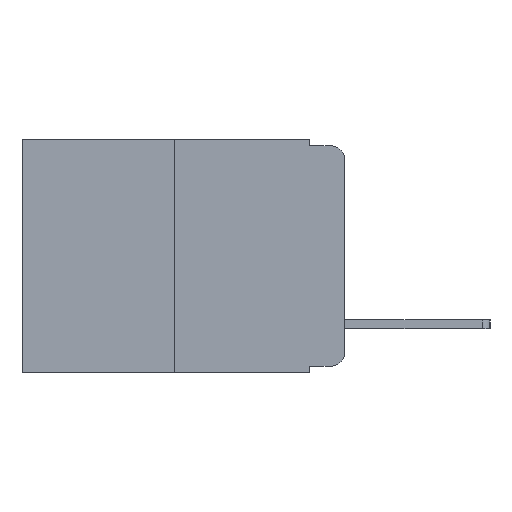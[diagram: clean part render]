
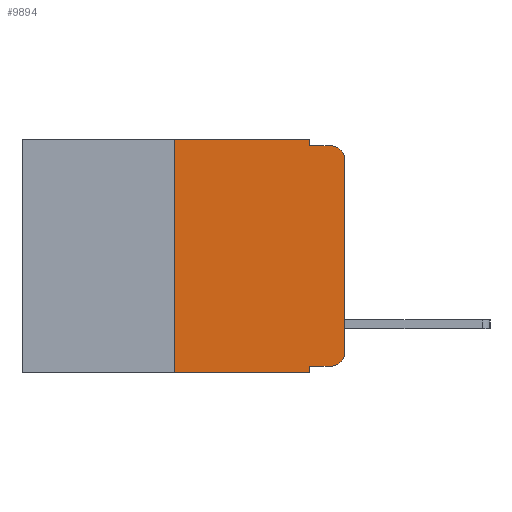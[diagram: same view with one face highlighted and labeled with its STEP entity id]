
A CAD part, left-side view. The second image highlights one B-rep face of the part: STEP entity #9894.
In plain terms, the highlighted planar face has unit normal (-1, 0, 0).
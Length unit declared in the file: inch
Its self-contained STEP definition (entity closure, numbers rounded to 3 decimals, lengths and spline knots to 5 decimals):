
#180 = ORIENTED_EDGE ( 'NONE', *, *, #7223, .T. ) ;
#393 = VERTEX_POINT ( 'NONE', #1976 ) ;
#436 = DIRECTION ( 'NONE',  ( -1., 0., 0. ) ) ;
#718 = CARTESIAN_POINT ( 'NONE',  ( 0., 0.25, 0. ) ) ;
#937 = AXIS2_PLACEMENT_3D ( 'NONE', #10834, #11770, #6180 ) ;
#984 = ORIENTED_EDGE ( 'NONE', *, *, #8508, .F. ) ;
#1038 = EDGE_CURVE ( 'NONE', #7669, #5206, #10918, .T. ) ;
#1183 = DIRECTION ( 'NONE',  ( 0., -1., 0. ) ) ;
#1198 = CARTESIAN_POINT ( 'NONE',  ( 0., 0.051, -0.01 ) ) ;
#1281 = DIRECTION ( 'NONE',  ( 0., -1., 0. ) ) ;
#1392 = LINE ( 'NONE', #8974, #8864 ) ;
#1441 = CARTESIAN_POINT ( 'NONE',  ( 0., 0.473, 0. ) ) ;
#1643 = DIRECTION ( 'NONE',  ( 0., 0., 1. ) ) ;
#1976 = CARTESIAN_POINT ( 'NONE',  ( 0., 0., -0.03 ) ) ;
#2035 = CARTESIAN_POINT ( 'NONE',  ( 0., 0.051, -0.01 ) ) ;
#2045 = VERTEX_POINT ( 'NONE', #6982 ) ;
#2068 = VERTEX_POINT ( 'NONE', #4722 ) ;
#2250 = ORIENTED_EDGE ( 'NONE', *, *, #1038, .F. ) ;
#2287 = ORIENTED_EDGE ( 'NONE', *, *, #7891, .T. ) ;
#2436 = EDGE_CURVE ( 'NONE', #393, #5206, #3619, .T. ) ;
#2439 = ORIENTED_EDGE ( 'NONE', *, *, #9096, .F. ) ;
#2883 = DIRECTION ( 'NONE',  ( 0., -1., 0. ) ) ;
#3076 = VECTOR ( 'NONE', #1183, 39.37008 ) ;
#3100 = EDGE_CURVE ( 'NONE', #3775, #393, #9310, .T. ) ;
#3619 = CIRCLE ( 'NONE', #5348, 0.02 ) ;
#3775 = VERTEX_POINT ( 'NONE', #7620 ) ;
#3866 = ORIENTED_EDGE ( 'NONE', *, *, #3100, .T. ) ;
#3903 = DIRECTION ( 'NONE',  ( 0., 0., -1. ) ) ;
#3988 = ORIENTED_EDGE ( 'NONE', *, *, #10944, .F. ) ;
#4083 = ORIENTED_EDGE ( 'NONE', *, *, #4863, .F. ) ;
#4165 = LINE ( 'NONE', #11394, #8971 ) ;
#4176 = ORIENTED_EDGE ( 'NONE', *, *, #11501, .T. ) ;
#4252 = ORIENTED_EDGE ( 'NONE', *, *, #2436, .T. ) ;
#4592 = VERTEX_POINT ( 'NONE', #7899 ) ;
#4722 = CARTESIAN_POINT ( 'NONE',  ( 0., 0.25, 0. ) ) ;
#4732 = CARTESIAN_POINT ( 'NONE',  ( 0., 0.473, -0.343 ) ) ;
#4863 = EDGE_CURVE ( 'NONE', #2068, #7177, #11222, .T. ) ;
#4869 = VECTOR ( 'NONE', #3903, 39.37008 ) ;
#5171 = PLANE ( 'NONE',  #937 ) ;
#5206 = VERTEX_POINT ( 'NONE', #6842 ) ;
#5252 = CARTESIAN_POINT ( 'NONE',  ( 0., 0.02, -0.313 ) ) ;
#5348 = AXIS2_PLACEMENT_3D ( 'NONE', #6390, #436, #7385 ) ;
#6058 = AXIS2_PLACEMENT_3D ( 'NONE', #5252, #11837, #6245 ) ;
#6180 = DIRECTION ( 'NONE',  ( 0., 0., -1. ) ) ;
#6240 = VECTOR ( 'NONE', #8288, 39.37008 ) ;
#6245 = DIRECTION ( 'NONE',  ( 0., 0., -1. ) ) ;
#6390 = CARTESIAN_POINT ( 'NONE',  ( 0., 0.02, -0.03 ) ) ;
#6752 = DIRECTION ( 'NONE',  ( 0., 0., -1. ) ) ;
#6823 = CARTESIAN_POINT ( 'NONE',  ( 0., 0.051, 0. ) ) ;
#6842 = CARTESIAN_POINT ( 'NONE',  ( 0., 0.02, -0.01 ) ) ;
#6982 = CARTESIAN_POINT ( 'NONE',  ( 0., 0.051, -0.333 ) ) ;
#7162 = LINE ( 'NONE', #6823, #4869 ) ;
#7177 = VERTEX_POINT ( 'NONE', #8075 ) ;
#7223 = EDGE_CURVE ( 'NONE', #4592, #3775, #10583, .T. ) ;
#7385 = DIRECTION ( 'NONE',  ( 0., 0., -1. ) ) ;
#7620 = CARTESIAN_POINT ( 'NONE',  ( 0., 0., -0.313 ) ) ;
#7669 = VERTEX_POINT ( 'NONE', #2035 ) ;
#7891 = EDGE_CURVE ( 'NONE', #2045, #4592, #1392, .T. ) ;
#7899 = CARTESIAN_POINT ( 'NONE',  ( 0., 0.02, -0.333 ) ) ;
#7961 = VECTOR ( 'NONE', #10417, 39.37008 ) ;
#8075 = CARTESIAN_POINT ( 'NONE',  ( 0., 0.051, 0. ) ) ;
#8288 = DIRECTION ( 'NONE',  ( 0., -1., 0. ) ) ;
#8340 = VERTEX_POINT ( 'NONE', #10227 ) ;
#8508 = EDGE_CURVE ( 'NONE', #2045, #8340, #4165, .T. ) ;
#8705 = VECTOR ( 'NONE', #2883, 39.37008 ) ;
#8864 = VECTOR ( 'NONE', #1281, 39.37008 ) ;
#8971 = VECTOR ( 'NONE', #6752, 39.37008 ) ;
#8974 = CARTESIAN_POINT ( 'NONE',  ( 0., 0.051, -0.333 ) ) ;
#8984 = VERTEX_POINT ( 'NONE', #10213 ) ;
#9096 = EDGE_CURVE ( 'NONE', #8984, #2068, #10386, .T. ) ;
#9310 = LINE ( 'NONE', #10193, #11470 ) ;
#9360 = FACE_OUTER_BOUND ( 'NONE', #10904, .T. ) ;
#9894 = ADVANCED_FACE ( 'NONE', ( #9360 ), #5171, .F. ) ;
#10193 = CARTESIAN_POINT ( 'NONE',  ( 0., 0., 0. ) ) ;
#10213 = CARTESIAN_POINT ( 'NONE',  ( 0., 0.25, -0.343 ) ) ;
#10227 = CARTESIAN_POINT ( 'NONE',  ( 0., 0.051, -0.343 ) ) ;
#10386 = LINE ( 'NONE', #718, #7961 ) ;
#10417 = DIRECTION ( 'NONE',  ( 0., 0., 1. ) ) ;
#10583 = CIRCLE ( 'NONE', #6058, 0.02 ) ;
#10834 = CARTESIAN_POINT ( 'NONE',  ( 0., 0.473, 0. ) ) ;
#10904 = EDGE_LOOP ( 'NONE', ( #3866, #4252, #2250, #3988, #4083, #2439, #4176, #984, #2287, #180 ) ) ;
#10918 = LINE ( 'NONE', #1198, #3076 ) ;
#10944 = EDGE_CURVE ( 'NONE', #7177, #7669, #7162, .T. ) ;
#11136 = LINE ( 'NONE', #4732, #8705 ) ;
#11222 = LINE ( 'NONE', #1441, #6240 ) ;
#11394 = CARTESIAN_POINT ( 'NONE',  ( 0., 0.051, 0. ) ) ;
#11470 = VECTOR ( 'NONE', #1643, 39.37008 ) ;
#11501 = EDGE_CURVE ( 'NONE', #8984, #8340, #11136, .T. ) ;
#11770 = DIRECTION ( 'NONE',  ( 1., 0., 0. ) ) ;
#11837 = DIRECTION ( 'NONE',  ( -1., 0., 0. ) ) ;
